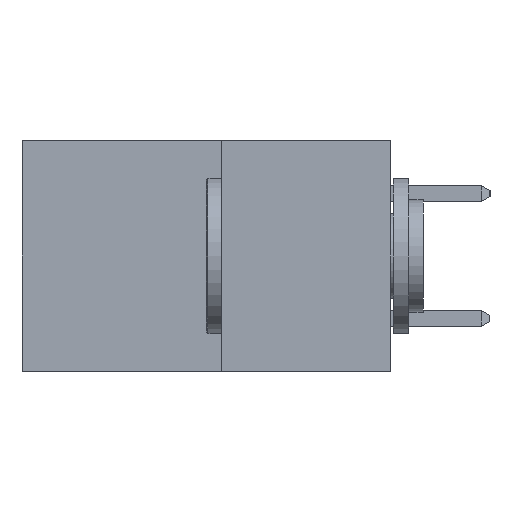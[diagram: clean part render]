
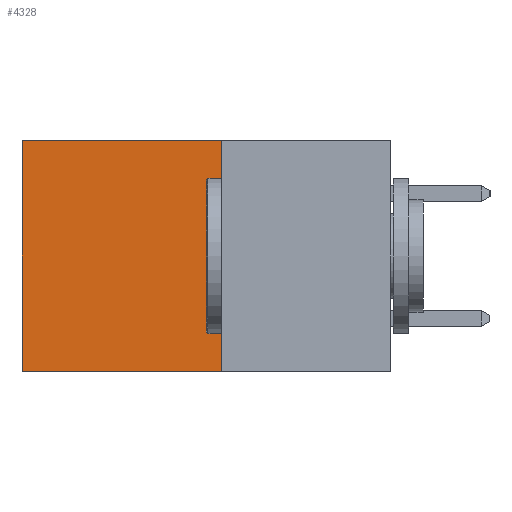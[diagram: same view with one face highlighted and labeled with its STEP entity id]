
A CAD part, left-side view. The second image highlights one B-rep face of the part: STEP entity #4328.
In plain terms, the highlighted planar face has unit normal (-1, 0, 0).
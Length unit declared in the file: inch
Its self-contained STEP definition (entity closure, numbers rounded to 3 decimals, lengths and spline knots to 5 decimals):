
#517 = LINE ( 'NONE', #2356, #2882 ) ;
#1046 = DIRECTION ( 'NONE',  ( 0., 1., 0. ) ) ;
#1620 = EDGE_CURVE ( 'NONE', #9024, #3079, #2136, .T. ) ;
#1878 = ORIENTED_EDGE ( 'NONE', *, *, #3064, .T. ) ;
#2136 = LINE ( 'NONE', #4602, #12342 ) ;
#2356 = CARTESIAN_POINT ( 'NONE',  ( 0.277, 0.27, 0. ) ) ;
#2882 = VECTOR ( 'NONE', #1046, 39.37008 ) ;
#2924 = DIRECTION ( 'NONE',  ( 0., 0., -1. ) ) ;
#3064 = EDGE_CURVE ( 'NONE', #11674, #3120, #12758, .T. ) ;
#3079 = VERTEX_POINT ( 'NONE', #9747 ) ;
#3120 = VERTEX_POINT ( 'NONE', #8607 ) ;
#4246 = CARTESIAN_POINT ( 'NONE',  ( 0.277, 0.59, -0.37 ) ) ;
#4323 = CARTESIAN_POINT ( 'NONE',  ( 0.277, 0.59, 0. ) ) ;
#4328 = ADVANCED_FACE ( 'NONE', ( #4874 ), #12337, .F. ) ;
#4602 = CARTESIAN_POINT ( 'NONE',  ( 0.277, 0.27, -0.37 ) ) ;
#4874 = FACE_OUTER_BOUND ( 'NONE', #8425, .T. ) ;
#5180 = ORIENTED_EDGE ( 'NONE', *, *, #1620, .F. ) ;
#7219 = CARTESIAN_POINT ( 'NONE',  ( 0.277, 0.27, 0. ) ) ;
#7303 = VECTOR ( 'NONE', #2924, 39.37008 ) ;
#8070 = DIRECTION ( 'NONE',  ( 0., 1., 0. ) ) ;
#8425 = EDGE_LOOP ( 'NONE', ( #1878, #12717, #5180, #10728 ) ) ;
#8607 = CARTESIAN_POINT ( 'NONE',  ( 0.277, 0.59, -0.37 ) ) ;
#9024 = VERTEX_POINT ( 'NONE', #7219 ) ;
#9747 = CARTESIAN_POINT ( 'NONE',  ( 0.277, 0.27, -0.37 ) ) ;
#9796 = AXIS2_PLACEMENT_3D ( 'NONE', #12958, #12894, #13074 ) ;
#9803 = VECTOR ( 'NONE', #8070, 39.37008 ) ;
#10131 = LINE ( 'NONE', #11178, #9803 ) ;
#10171 = EDGE_CURVE ( 'NONE', #9024, #11674, #517, .T. ) ;
#10193 = DIRECTION ( 'NONE',  ( 0., 0., -1. ) ) ;
#10728 = ORIENTED_EDGE ( 'NONE', *, *, #10171, .T. ) ;
#11178 = CARTESIAN_POINT ( 'NONE',  ( 0.277, 0.27, -0.37 ) ) ;
#11453 = EDGE_CURVE ( 'NONE', #3079, #3120, #10131, .T. ) ;
#11674 = VERTEX_POINT ( 'NONE', #4323 ) ;
#12337 = PLANE ( 'NONE',  #9796 ) ;
#12342 = VECTOR ( 'NONE', #10193, 39.37008 ) ;
#12717 = ORIENTED_EDGE ( 'NONE', *, *, #11453, .F. ) ;
#12758 = LINE ( 'NONE', #4246, #7303 ) ;
#12894 = DIRECTION ( 'NONE',  ( 1., 0., 0. ) ) ;
#12958 = CARTESIAN_POINT ( 'NONE',  ( 0.277, 0.27, -0.37 ) ) ;
#13074 = DIRECTION ( 'NONE',  ( 0., 0., -1. ) ) ;
